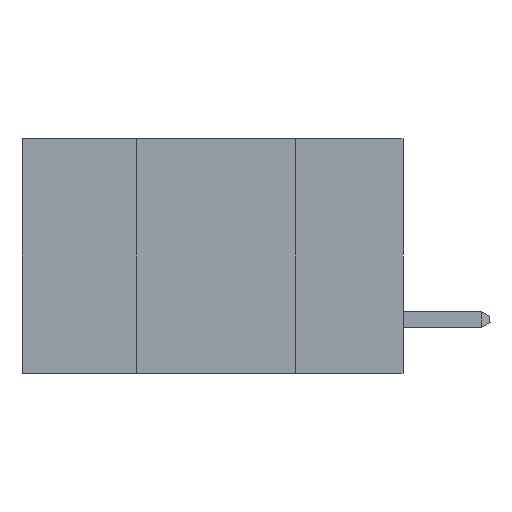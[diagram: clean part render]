
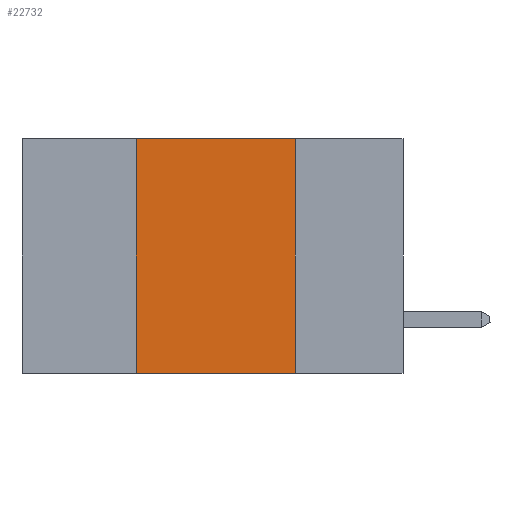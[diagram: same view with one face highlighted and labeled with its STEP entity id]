
A CAD part, left-side view. The second image highlights one B-rep face of the part: STEP entity #22732.
In plain terms, the highlighted planar face has unit normal (-1, 0, 0).
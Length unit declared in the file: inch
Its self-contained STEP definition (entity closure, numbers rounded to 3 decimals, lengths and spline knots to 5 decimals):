
#767 = ORIENTED_EDGE ( 'NONE', *, *, #10148, .F. ) ;
#1131 = LINE ( 'NONE', #11497, #32238 ) ;
#1174 = CARTESIAN_POINT ( 'NONE',  ( 0., 0.42, 0. ) ) ;
#3375 = AXIS2_PLACEMENT_3D ( 'NONE', #18057, #10188, #31547 ) ;
#5213 = VERTEX_POINT ( 'NONE', #1174 ) ;
#5790 = CARTESIAN_POINT ( 'NONE',  ( 0., 0.42, -0.37 ) ) ;
#6430 = CARTESIAN_POINT ( 'NONE',  ( 0., 0.6, -0.37 ) ) ;
#6857 = VERTEX_POINT ( 'NONE', #33693 ) ;
#7256 = LINE ( 'NONE', #17575, #22312 ) ;
#8447 = VERTEX_POINT ( 'NONE', #31211 ) ;
#10148 = EDGE_CURVE ( 'NONE', #5213, #8447, #1131, .T. ) ;
#10188 = DIRECTION ( 'NONE',  ( 1., 0., 0. ) ) ;
#10972 = LINE ( 'NONE', #6430, #31164 ) ;
#11497 = CARTESIAN_POINT ( 'NONE',  ( 0., 0.6, 0. ) ) ;
#12600 = EDGE_CURVE ( 'NONE', #14263, #6857, #10972, .T. ) ;
#14263 = VERTEX_POINT ( 'NONE', #5790 ) ;
#17341 = DIRECTION ( 'NONE',  ( 0., 0., -1. ) ) ;
#17560 = ORIENTED_EDGE ( 'NONE', *, *, #12600, .T. ) ;
#17575 = CARTESIAN_POINT ( 'NONE',  ( 0., 0.17, 0. ) ) ;
#17793 = EDGE_LOOP ( 'NONE', ( #18544, #767, #26793, #17560 ) ) ;
#17826 = PLANE ( 'NONE',  #3375 ) ;
#18057 = CARTESIAN_POINT ( 'NONE',  ( 0., 0.6, 0. ) ) ;
#18402 = EDGE_CURVE ( 'NONE', #14263, #5213, #28166, .T. ) ;
#18544 = ORIENTED_EDGE ( 'NONE', *, *, #20761, .F. ) ;
#20761 = EDGE_CURVE ( 'NONE', #8447, #6857, #7256, .T. ) ;
#22312 = VECTOR ( 'NONE', #17341, 39.37008 ) ;
#22732 = ADVANCED_FACE ( 'NONE', ( #25143 ), #17826, .F. ) ;
#25143 = FACE_OUTER_BOUND ( 'NONE', #17793, .T. ) ;
#26793 = ORIENTED_EDGE ( 'NONE', *, *, #18402, .F. ) ;
#27319 = VECTOR ( 'NONE', #29261, 39.37008 ) ;
#28166 = LINE ( 'NONE', #34402, #27319 ) ;
#29128 = DIRECTION ( 'NONE',  ( 0., -1., 0. ) ) ;
#29261 = DIRECTION ( 'NONE',  ( 0., 0., 1. ) ) ;
#31164 = VECTOR ( 'NONE', #33179, 39.37008 ) ;
#31211 = CARTESIAN_POINT ( 'NONE',  ( 0., 0.17, 0. ) ) ;
#31547 = DIRECTION ( 'NONE',  ( 0., 0., -1. ) ) ;
#32238 = VECTOR ( 'NONE', #29128, 39.37008 ) ;
#33179 = DIRECTION ( 'NONE',  ( 0., -1., 0. ) ) ;
#33693 = CARTESIAN_POINT ( 'NONE',  ( 0., 0.17, -0.37 ) ) ;
#34402 = CARTESIAN_POINT ( 'NONE',  ( 0., 0.42, 0. ) ) ;
